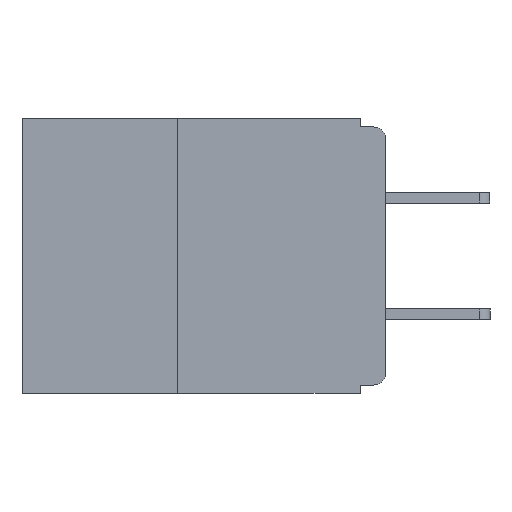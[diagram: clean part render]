
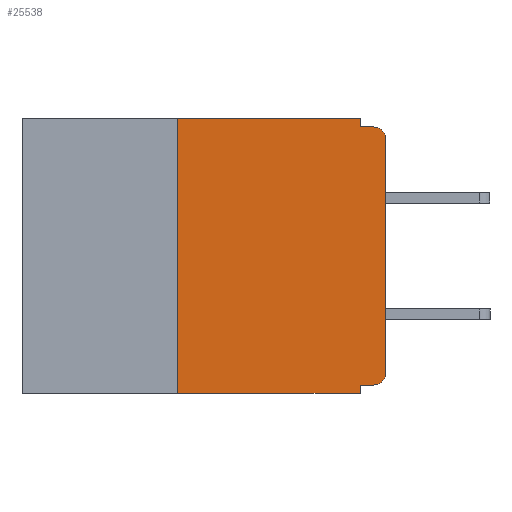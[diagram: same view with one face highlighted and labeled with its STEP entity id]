
A CAD part, left-side view. The second image highlights one B-rep face of the part: STEP entity #25538.
In plain terms, the highlighted planar face has unit normal (-1, 0, 0).
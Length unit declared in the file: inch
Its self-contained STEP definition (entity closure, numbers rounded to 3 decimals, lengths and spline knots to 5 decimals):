
#52 = EDGE_CURVE ( 'NONE', #6884, #16950, #6590, .T. ) ;
#153 = LINE ( 'NONE', #23384, #22302 ) ;
#204 = VERTEX_POINT ( 'NONE', #14876 ) ;
#878 = ORIENTED_EDGE ( 'NONE', *, *, #24831, .F. ) ;
#1104 = VERTEX_POINT ( 'NONE', #9192 ) ;
#1163 = DIRECTION ( 'NONE',  ( 0., 1., 0. ) ) ;
#1453 = VERTEX_POINT ( 'NONE', #23922 ) ;
#1525 = DIRECTION ( 'NONE',  ( 0., 0., 1. ) ) ;
#1554 = CARTESIAN_POINT ( 'NONE',  ( 0., 0., -0.32 ) ) ;
#1929 = CARTESIAN_POINT ( 'NONE',  ( 0., 0.437, 0. ) ) ;
#2031 = DIRECTION ( 'NONE',  ( 0., 0., -1. ) ) ;
#2599 = CARTESIAN_POINT ( 'NONE',  ( 0., 0.031, 0. ) ) ;
#2755 = EDGE_CURVE ( 'NONE', #1453, #25712, #13464, .T. ) ;
#2996 = ORIENTED_EDGE ( 'NONE', *, *, #21144, .F. ) ;
#3110 = ORIENTED_EDGE ( 'NONE', *, *, #24580, .F. ) ;
#3178 = ORIENTED_EDGE ( 'NONE', *, *, #5160, .F. ) ;
#3528 = LINE ( 'NONE', #2599, #8557 ) ;
#3913 = EDGE_CURVE ( 'NONE', #18326, #5951, #25957, .T. ) ;
#4138 = ORIENTED_EDGE ( 'NONE', *, *, #3913, .T. ) ;
#4463 = ORIENTED_EDGE ( 'NONE', *, *, #9314, .F. ) ;
#4758 = CARTESIAN_POINT ( 'NONE',  ( 0., 0.437, 0. ) ) ;
#4919 = VECTOR ( 'NONE', #26450, 39.37008 ) ;
#4983 = ORIENTED_EDGE ( 'NONE', *, *, #6482, .F. ) ;
#5160 = EDGE_CURVE ( 'NONE', #18326, #204, #153, .T. ) ;
#5162 = CARTESIAN_POINT ( 'NONE',  ( 0., 0.25, -0.33 ) ) ;
#5518 = VERTEX_POINT ( 'NONE', #27007 ) ;
#5663 = VECTOR ( 'NONE', #17519, 39.37008 ) ;
#5878 = ORIENTED_EDGE ( 'NONE', *, *, #2755, .T. ) ;
#5901 = LINE ( 'NONE', #14467, #10898 ) ;
#5951 = VERTEX_POINT ( 'NONE', #16880 ) ;
#6482 = EDGE_CURVE ( 'NONE', #1453, #13696, #9377, .T. ) ;
#6590 = CIRCLE ( 'NONE', #18519, 0.015 ) ;
#6884 = VERTEX_POINT ( 'NONE', #13746 ) ;
#6889 = CARTESIAN_POINT ( 'NONE',  ( 0., 0.015, -0.025 ) ) ;
#8217 = DIRECTION ( 'NONE',  ( 0., -1., 0. ) ) ;
#8393 = DIRECTION ( 'NONE',  ( -1., 0., 0. ) ) ;
#8557 = VECTOR ( 'NONE', #19714, 39.37008 ) ;
#8701 = VECTOR ( 'NONE', #1163, 39.37008 ) ;
#9083 = VECTOR ( 'NONE', #12326, 39.37008 ) ;
#9192 = CARTESIAN_POINT ( 'NONE',  ( 0., 0.031, 0. ) ) ;
#9314 = EDGE_CURVE ( 'NONE', #13696, #5951, #26736, .T. ) ;
#9377 = LINE ( 'NONE', #1554, #8701 ) ;
#9920 = FACE_OUTER_BOUND ( 'NONE', #15839, .T. ) ;
#9925 = CARTESIAN_POINT ( 'NONE',  ( 0., 0.437, -0.33 ) ) ;
#10613 = PLANE ( 'NONE',  #22085 ) ;
#10898 = VECTOR ( 'NONE', #1525, 39.37008 ) ;
#11308 = LINE ( 'NONE', #4758, #5663 ) ;
#12244 = DIRECTION ( 'NONE',  ( -1., 0., 0. ) ) ;
#12326 = DIRECTION ( 'NONE',  ( 0., -1., 0. ) ) ;
#13464 = CIRCLE ( 'NONE', #15239, 0.015 ) ;
#13637 = CARTESIAN_POINT ( 'NONE',  ( 0., 0.015, -0.01 ) ) ;
#13696 = VERTEX_POINT ( 'NONE', #22777 ) ;
#13746 = CARTESIAN_POINT ( 'NONE',  ( 0., 0., -0.025 ) ) ;
#14467 = CARTESIAN_POINT ( 'NONE',  ( 0., 0., 0. ) ) ;
#14876 = CARTESIAN_POINT ( 'NONE',  ( 0., 0.25, 0. ) ) ;
#14940 = DIRECTION ( 'NONE',  ( 1., 0., 0. ) ) ;
#15239 = AXIS2_PLACEMENT_3D ( 'NONE', #27431, #12244, #21238 ) ;
#15839 = EDGE_LOOP ( 'NONE', ( #23516, #26708, #878, #2996, #3110, #3178, #4138, #4463, #4983, #5878 ) ) ;
#16654 = LINE ( 'NONE', #27114, #26496 ) ;
#16822 = DIRECTION ( 'NONE',  ( 0., 0., -1. ) ) ;
#16880 = CARTESIAN_POINT ( 'NONE',  ( 0., 0.031, -0.33 ) ) ;
#16950 = VERTEX_POINT ( 'NONE', #13637 ) ;
#17519 = DIRECTION ( 'NONE',  ( 0., -1., 0. ) ) ;
#18326 = VERTEX_POINT ( 'NONE', #5162 ) ;
#18519 = AXIS2_PLACEMENT_3D ( 'NONE', #6889, #8393, #16822 ) ;
#19714 = DIRECTION ( 'NONE',  ( 0., 0., -1. ) ) ;
#19799 = CARTESIAN_POINT ( 'NONE',  ( 0., 0., -0.305 ) ) ;
#20846 = EDGE_CURVE ( 'NONE', #25712, #6884, #5901, .T. ) ;
#21144 = EDGE_CURVE ( 'NONE', #1104, #5518, #3528, .T. ) ;
#21238 = DIRECTION ( 'NONE',  ( 0., 0., -1. ) ) ;
#21787 = DIRECTION ( 'NONE',  ( 0., 0., 1. ) ) ;
#22085 = AXIS2_PLACEMENT_3D ( 'NONE', #1929, #14940, #2031 ) ;
#22302 = VECTOR ( 'NONE', #21787, 39.37008 ) ;
#22777 = CARTESIAN_POINT ( 'NONE',  ( 0., 0.031, -0.32 ) ) ;
#23384 = CARTESIAN_POINT ( 'NONE',  ( 0., 0.25, -0.33 ) ) ;
#23516 = ORIENTED_EDGE ( 'NONE', *, *, #20846, .T. ) ;
#23922 = CARTESIAN_POINT ( 'NONE',  ( 0., 0.015, -0.32 ) ) ;
#24580 = EDGE_CURVE ( 'NONE', #204, #1104, #11308, .T. ) ;
#24831 = EDGE_CURVE ( 'NONE', #5518, #16950, #16654, .T. ) ;
#25538 = ADVANCED_FACE ( 'NONE', ( #9920 ), #10613, .F. ) ;
#25712 = VERTEX_POINT ( 'NONE', #19799 ) ;
#25957 = LINE ( 'NONE', #9925, #9083 ) ;
#26450 = DIRECTION ( 'NONE',  ( 0., 0., -1. ) ) ;
#26496 = VECTOR ( 'NONE', #8217, 39.37008 ) ;
#26708 = ORIENTED_EDGE ( 'NONE', *, *, #52, .T. ) ;
#26736 = LINE ( 'NONE', #26948, #4919 ) ;
#26948 = CARTESIAN_POINT ( 'NONE',  ( 0., 0.031, -0.33 ) ) ;
#27007 = CARTESIAN_POINT ( 'NONE',  ( 0., 0.031, -0.01 ) ) ;
#27114 = CARTESIAN_POINT ( 'NONE',  ( 0., 0., -0.01 ) ) ;
#27431 = CARTESIAN_POINT ( 'NONE',  ( 0., 0.015, -0.305 ) ) ;
